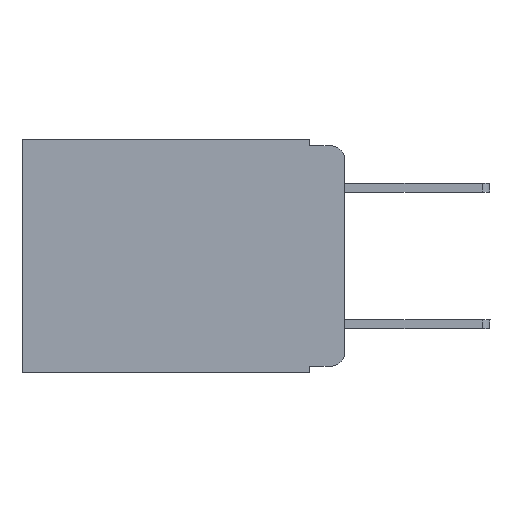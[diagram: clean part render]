
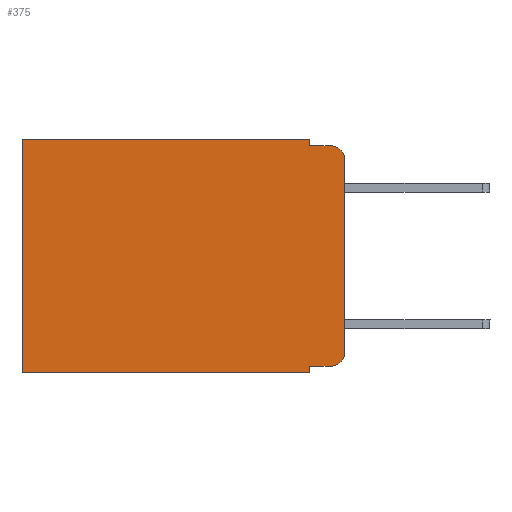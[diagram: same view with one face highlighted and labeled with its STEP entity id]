
A CAD part, left-side view. The second image highlights one B-rep face of the part: STEP entity #375.
In plain terms, the highlighted planar face has unit normal (-1, 0, 0).
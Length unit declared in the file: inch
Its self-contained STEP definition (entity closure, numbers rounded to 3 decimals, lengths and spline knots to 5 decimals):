
#280 = CARTESIAN_POINT ( 'NONE',  ( 0.298, 0., -0.03 ) ) ;
#375 = ADVANCED_FACE ( 'NONE', ( #6240 ), #3697, .F. ) ;
#382 = VERTEX_POINT ( 'NONE', #4937 ) ;
#515 = CARTESIAN_POINT ( 'NONE',  ( 0.298, 0.02, -0.333 ) ) ;
#721 = DIRECTION ( 'NONE',  ( -1., 0., 0. ) ) ;
#949 = DIRECTION ( 'NONE',  ( 0., 0., -1. ) ) ;
#1451 = VECTOR ( 'NONE', #9820, 39.37008 ) ;
#1504 = VERTEX_POINT ( 'NONE', #13031 ) ;
#1561 = EDGE_CURVE ( 'NONE', #382, #12836, #15765, .T. ) ;
#1847 = EDGE_CURVE ( 'NONE', #5315, #7686, #7791, .T. ) ;
#2902 = VECTOR ( 'NONE', #3116, 39.37008 ) ;
#2986 = DIRECTION ( 'NONE',  ( 0., -1., 0. ) ) ;
#3116 = DIRECTION ( 'NONE',  ( 0., 1., 0. ) ) ;
#3203 = EDGE_CURVE ( 'NONE', #6028, #5315, #13167, .T. ) ;
#3320 = AXIS2_PLACEMENT_3D ( 'NONE', #9643, #721, #5907 ) ;
#3504 = DIRECTION ( 'NONE',  ( 0., 0., -1. ) ) ;
#3610 = LINE ( 'NONE', #7466, #4633 ) ;
#3622 = EDGE_CURVE ( 'NONE', #5852, #1504, #8293, .T. ) ;
#3697 = PLANE ( 'NONE',  #14723 ) ;
#3974 = ORIENTED_EDGE ( 'NONE', *, *, #6519, .F. ) ;
#4304 = CARTESIAN_POINT ( 'NONE',  ( 0.298, 0., -0.313 ) ) ;
#4479 = LINE ( 'NONE', #8584, #1451 ) ;
#4584 = EDGE_LOOP ( 'NONE', ( #3974, #5927, #13294, #11799, #5504, #10548, #11751, #10562, #11459, #8319 ) ) ;
#4633 = VECTOR ( 'NONE', #5971, 39.37008 ) ;
#4736 = CARTESIAN_POINT ( 'NONE',  ( 0.298, 0.02, -0.03 ) ) ;
#4892 = VECTOR ( 'NONE', #9969, 39.37008 ) ;
#4931 = CARTESIAN_POINT ( 'NONE',  ( 0.298, 0.051, 0. ) ) ;
#4937 = CARTESIAN_POINT ( 'NONE',  ( 0.298, 0.051, -0.343 ) ) ;
#5315 = VERTEX_POINT ( 'NONE', #515 ) ;
#5504 = ORIENTED_EDGE ( 'NONE', *, *, #15201, .T. ) ;
#5741 = CARTESIAN_POINT ( 'NONE',  ( 0.298, 0.051, -0.01 ) ) ;
#5852 = VERTEX_POINT ( 'NONE', #9758 ) ;
#5872 = EDGE_CURVE ( 'NONE', #11075, #1504, #8479, .T. ) ;
#5907 = DIRECTION ( 'NONE',  ( 0., 0., -1. ) ) ;
#5927 = ORIENTED_EDGE ( 'NONE', *, *, #5872, .T. ) ;
#5939 = DIRECTION ( 'NONE',  ( -1., 0., 0. ) ) ;
#5971 = DIRECTION ( 'NONE',  ( 0., 0., -1. ) ) ;
#6028 = VERTEX_POINT ( 'NONE', #14558 ) ;
#6240 = FACE_OUTER_BOUND ( 'NONE', #4584, .T. ) ;
#6519 = EDGE_CURVE ( 'NONE', #11075, #7686, #11291, .T. ) ;
#6887 = VERTEX_POINT ( 'NONE', #6957 ) ;
#6957 = CARTESIAN_POINT ( 'NONE',  ( 0.298, 0.473, 0. ) ) ;
#7090 = LINE ( 'NONE', #13396, #11239 ) ;
#7293 = CARTESIAN_POINT ( 'NONE',  ( 0.298, 0.473, -0.343 ) ) ;
#7466 = CARTESIAN_POINT ( 'NONE',  ( 0.298, 0.051, 0. ) ) ;
#7686 = VERTEX_POINT ( 'NONE', #4304 ) ;
#7791 = CIRCLE ( 'NONE', #3320, 0.02 ) ;
#8164 = CARTESIAN_POINT ( 'NONE',  ( 0.298, 0.051, -0.333 ) ) ;
#8180 = CARTESIAN_POINT ( 'NONE',  ( 0.298, 0.473, 0. ) ) ;
#8293 = LINE ( 'NONE', #5741, #10380 ) ;
#8319 = ORIENTED_EDGE ( 'NONE', *, *, #1847, .T. ) ;
#8407 = VERTEX_POINT ( 'NONE', #4931 ) ;
#8479 = CIRCLE ( 'NONE', #10854, 0.02 ) ;
#8584 = CARTESIAN_POINT ( 'NONE',  ( 0.298, 0., 0. ) ) ;
#9235 = EDGE_CURVE ( 'NONE', #8407, #5852, #7090, .T. ) ;
#9536 = DIRECTION ( 'NONE',  ( 0., -1., 0. ) ) ;
#9643 = CARTESIAN_POINT ( 'NONE',  ( 0.298, 0.02, -0.313 ) ) ;
#9758 = CARTESIAN_POINT ( 'NONE',  ( 0.298, 0.051, -0.01 ) ) ;
#9820 = DIRECTION ( 'NONE',  ( 0., 1., 0. ) ) ;
#9871 = DIRECTION ( 'NONE',  ( 1., 0., 0. ) ) ;
#9969 = DIRECTION ( 'NONE',  ( 0., 0., -1. ) ) ;
#10035 = CARTESIAN_POINT ( 'NONE',  ( 0.298, 0., 0. ) ) ;
#10380 = VECTOR ( 'NONE', #9536, 39.37008 ) ;
#10548 = ORIENTED_EDGE ( 'NONE', *, *, #12917, .T. ) ;
#10562 = ORIENTED_EDGE ( 'NONE', *, *, #16175, .F. ) ;
#10854 = AXIS2_PLACEMENT_3D ( 'NONE', #4736, #5939, #13489 ) ;
#11075 = VERTEX_POINT ( 'NONE', #280 ) ;
#11239 = VECTOR ( 'NONE', #12146, 39.37008 ) ;
#11291 = LINE ( 'NONE', #12784, #4892 ) ;
#11459 = ORIENTED_EDGE ( 'NONE', *, *, #3203, .T. ) ;
#11751 = ORIENTED_EDGE ( 'NONE', *, *, #1561, .F. ) ;
#11799 = ORIENTED_EDGE ( 'NONE', *, *, #9235, .F. ) ;
#12146 = DIRECTION ( 'NONE',  ( 0., 0., -1. ) ) ;
#12784 = CARTESIAN_POINT ( 'NONE',  ( 0.298, 0., 0. ) ) ;
#12836 = VERTEX_POINT ( 'NONE', #7293 ) ;
#12917 = EDGE_CURVE ( 'NONE', #6887, #12836, #14492, .T. ) ;
#13031 = CARTESIAN_POINT ( 'NONE',  ( 0.298, 0.02, -0.01 ) ) ;
#13164 = VECTOR ( 'NONE', #2986, 39.37008 ) ;
#13167 = LINE ( 'NONE', #8164, #13164 ) ;
#13294 = ORIENTED_EDGE ( 'NONE', *, *, #3622, .F. ) ;
#13396 = CARTESIAN_POINT ( 'NONE',  ( 0.298, 0.051, 0. ) ) ;
#13450 = CARTESIAN_POINT ( 'NONE',  ( 0.298, 0., -0.343 ) ) ;
#13489 = DIRECTION ( 'NONE',  ( 0., 0., -1. ) ) ;
#14492 = LINE ( 'NONE', #8180, #15908 ) ;
#14558 = CARTESIAN_POINT ( 'NONE',  ( 0.298, 0.051, -0.333 ) ) ;
#14723 = AXIS2_PLACEMENT_3D ( 'NONE', #10035, #9871, #949 ) ;
#15201 = EDGE_CURVE ( 'NONE', #8407, #6887, #4479, .T. ) ;
#15765 = LINE ( 'NONE', #13450, #2902 ) ;
#15908 = VECTOR ( 'NONE', #3504, 39.37008 ) ;
#16175 = EDGE_CURVE ( 'NONE', #6028, #382, #3610, .T. ) ;
